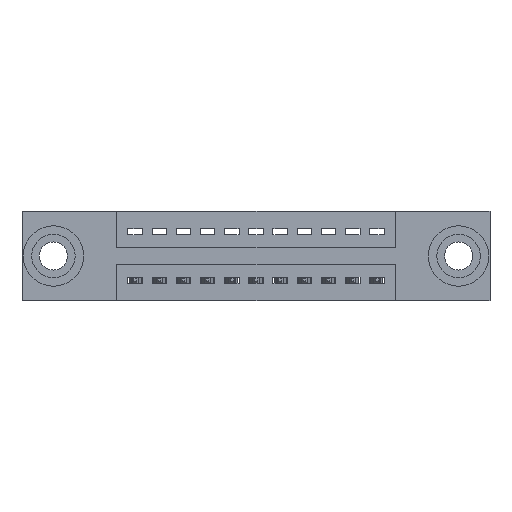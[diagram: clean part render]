
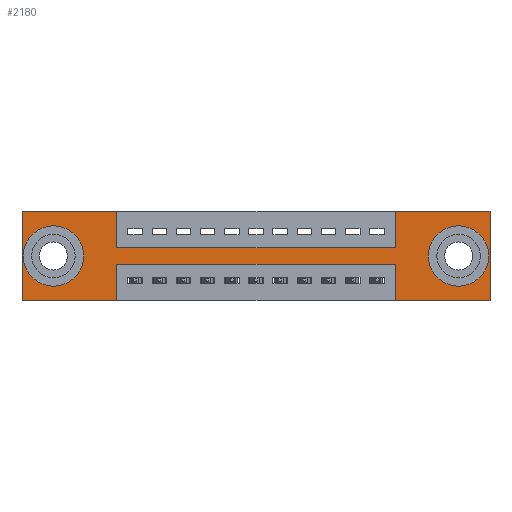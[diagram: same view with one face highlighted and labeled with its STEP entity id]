
A CAD part, front view. The second image highlights one B-rep face of the part: STEP entity #2180.
In plain terms, the highlighted planar face has unit normal (0, -1, 0).
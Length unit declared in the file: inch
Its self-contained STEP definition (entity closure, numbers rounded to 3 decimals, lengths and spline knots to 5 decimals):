
#14 = ORIENTED_EDGE ( 'NONE', *, *, #1394, .T. ) ;
#212 = CARTESIAN_POINT ( 'NONE',  ( 0., 0., 0. ) ) ;
#308 = DIRECTION ( 'NONE',  ( 1., 0., 0. ) ) ;
#668 = EDGE_CURVE ( 'NONE', #12235, #11286, #8197, .T. ) ;
#871 = CARTESIAN_POINT ( 'NONE',  ( 0., 0., 0. ) ) ;
#1046 = CARTESIAN_POINT ( 'NONE',  ( 1.805, 0., -0.185 ) ) ;
#1099 = DIRECTION ( 'NONE',  ( 0., 0., -1. ) ) ;
#1185 = VERTEX_POINT ( 'NONE', #2529 ) ;
#1215 = VERTEX_POINT ( 'NONE', #10645 ) ;
#1394 = EDGE_CURVE ( 'NONE', #10542, #4427, #11053, .T. ) ;
#1672 = VERTEX_POINT ( 'NONE', #3221 ) ;
#1677 = ORIENTED_EDGE ( 'NONE', *, *, #7910, .F. ) ;
#1680 = VERTEX_POINT ( 'NONE', #9301 ) ;
#1684 = EDGE_CURVE ( 'NONE', #12751, #1672, #8982, .T. ) ;
#1815 = DIRECTION ( 'NONE',  ( -1., 0., 0. ) ) ;
#1883 = FACE_BOUND ( 'NONE', #3871, .T. ) ;
#2007 = EDGE_CURVE ( 'NONE', #8037, #3869, #12929, .T. ) ;
#2175 = ORIENTED_EDGE ( 'NONE', *, *, #5121, .F. ) ;
#2180 = ADVANCED_FACE ( 'NONE', ( #1883, #2492, #6230 ), #6213, .T. ) ;
#2492 = FACE_BOUND ( 'NONE', #5449, .T. ) ;
#2529 = CARTESIAN_POINT ( 'NONE',  ( 1.5425, 0., -0.37 ) ) ;
#2872 = VERTEX_POINT ( 'NONE', #11516 ) ;
#2960 = LINE ( 'NONE', #13005, #7366 ) ;
#3043 = LINE ( 'NONE', #7125, #10966 ) ;
#3183 = VECTOR ( 'NONE', #3648, 39.37008 ) ;
#3221 = CARTESIAN_POINT ( 'NONE',  ( 0.3925, 0., 0. ) ) ;
#3309 = CARTESIAN_POINT ( 'NONE',  ( 0., 0., -0.37 ) ) ;
#3332 = DIRECTION ( 'NONE',  ( 0., 0., 1. ) ) ;
#3648 = DIRECTION ( 'NONE',  ( 0., 0., 1. ) ) ;
#3706 = VECTOR ( 'NONE', #9759, 39.37008 ) ;
#3869 = VERTEX_POINT ( 'NONE', #5413 ) ;
#3871 = EDGE_LOOP ( 'NONE', ( #14, #8239 ) ) ;
#4100 = ORIENTED_EDGE ( 'NONE', *, *, #7931, .F. ) ;
#4155 = LINE ( 'NONE', #871, #3706 ) ;
#4224 = DIRECTION ( 'NONE',  ( 1., 0., 0. ) ) ;
#4356 = ORIENTED_EDGE ( 'NONE', *, *, #10420, .F. ) ;
#4414 = ORIENTED_EDGE ( 'NONE', *, *, #11345, .F. ) ;
#4427 = VERTEX_POINT ( 'NONE', #6803 ) ;
#4953 = CARTESIAN_POINT ( 'NONE',  ( 1.805, 0., -0.107 ) ) ;
#5121 = EDGE_CURVE ( 'NONE', #1185, #5389, #6122, .T. ) ;
#5202 = CARTESIAN_POINT ( 'NONE',  ( 0., 0., -0.37 ) ) ;
#5235 = CIRCLE ( 'NONE', #8887, 0.078 ) ;
#5389 = VERTEX_POINT ( 'NONE', #5481 ) ;
#5399 = VERTEX_POINT ( 'NONE', #3309 ) ;
#5413 = CARTESIAN_POINT ( 'NONE',  ( 1.5425, 0., 0. ) ) ;
#5449 = EDGE_LOOP ( 'NONE', ( #11569, #8140 ) ) ;
#5481 = CARTESIAN_POINT ( 'NONE',  ( 1.5425, 0., -0.22 ) ) ;
#5572 = AXIS2_PLACEMENT_3D ( 'NONE', #1046, #8006, #12036 ) ;
#5730 = EDGE_CURVE ( 'NONE', #5399, #12751, #7099, .T. ) ;
#5786 = VECTOR ( 'NONE', #12247, 39.37008 ) ;
#5920 = CARTESIAN_POINT ( 'NONE',  ( 1.935, 0., 0. ) ) ;
#5929 = LINE ( 'NONE', #9885, #6879 ) ;
#5991 = VERTEX_POINT ( 'NONE', #11197 ) ;
#6013 = CARTESIAN_POINT ( 'NONE',  ( 1.5425, 0., -0.15 ) ) ;
#6081 = EDGE_CURVE ( 'NONE', #4427, #10542, #12952, .T. ) ;
#6113 = DIRECTION ( 'NONE',  ( 0., 0., 1. ) ) ;
#6122 = LINE ( 'NONE', #9757, #3183 ) ;
#6207 = LINE ( 'NONE', #5920, #11648 ) ;
#6213 = PLANE ( 'NONE',  #9768 ) ;
#6230 = FACE_OUTER_BOUND ( 'NONE', #8452, .T. ) ;
#6234 = DIRECTION ( 'NONE',  ( 0., 0., -1. ) ) ;
#6285 = DIRECTION ( 'NONE',  ( 0., 1., 0. ) ) ;
#6645 = EDGE_CURVE ( 'NONE', #2872, #8037, #8993, .T. ) ;
#6803 = CARTESIAN_POINT ( 'NONE',  ( 1.805, 0., -0.263 ) ) ;
#6879 = VECTOR ( 'NONE', #8748, 39.37008 ) ;
#6917 = DIRECTION ( 'NONE',  ( -1., 0., 0. ) ) ;
#7029 = VECTOR ( 'NONE', #6917, 39.37008 ) ;
#7099 = LINE ( 'NONE', #8127, #7906 ) ;
#7125 = CARTESIAN_POINT ( 'NONE',  ( 0.3925, 0., 0. ) ) ;
#7149 = CARTESIAN_POINT ( 'NONE',  ( 1.805, 0., -0.185 ) ) ;
#7234 = CARTESIAN_POINT ( 'NONE',  ( 0.3925, 0., -0.15 ) ) ;
#7257 = DIRECTION ( 'NONE',  ( 0., 0., -1. ) ) ;
#7366 = VECTOR ( 'NONE', #1815, 39.37008 ) ;
#7759 = AXIS2_PLACEMENT_3D ( 'NONE', #7149, #10993, #6234 ) ;
#7906 = VECTOR ( 'NONE', #6113, 39.37008 ) ;
#7910 = EDGE_CURVE ( 'NONE', #11834, #5399, #2960, .T. ) ;
#7931 = EDGE_CURVE ( 'NONE', #5389, #5991, #9746, .T. ) ;
#8006 = DIRECTION ( 'NONE',  ( 0., 1., 0. ) ) ;
#8021 = VECTOR ( 'NONE', #308, 39.37008 ) ;
#8037 = VERTEX_POINT ( 'NONE', #6013 ) ;
#8086 = CARTESIAN_POINT ( 'NONE',  ( 0., 0., -0.37 ) ) ;
#8127 = CARTESIAN_POINT ( 'NONE',  ( 0., 0., 0. ) ) ;
#8140 = ORIENTED_EDGE ( 'NONE', *, *, #668, .T. ) ;
#8197 = CIRCLE ( 'NONE', #12876, 0.078 ) ;
#8239 = ORIENTED_EDGE ( 'NONE', *, *, #6081, .T. ) ;
#8273 = CARTESIAN_POINT ( 'NONE',  ( 0., 0., 0. ) ) ;
#8284 = LINE ( 'NONE', #5202, #8777 ) ;
#8409 = CARTESIAN_POINT ( 'NONE',  ( 0.13, 0., -0.185 ) ) ;
#8452 = EDGE_LOOP ( 'NONE', ( #4356, #4100, #2175, #12568, #4414, #11781, #12353, #9204, #8697, #11419, #12489, #1677 ) ) ;
#8485 = CARTESIAN_POINT ( 'NONE',  ( 0.3925, 0., -0.37 ) ) ;
#8697 = ORIENTED_EDGE ( 'NONE', *, *, #12548, .F. ) ;
#8748 = DIRECTION ( 'NONE',  ( 0., 0., -1. ) ) ;
#8777 = VECTOR ( 'NONE', #10359, 39.37008 ) ;
#8875 = CARTESIAN_POINT ( 'NONE',  ( 0.13, 0., -0.107 ) ) ;
#8887 = AXIS2_PLACEMENT_3D ( 'NONE', #10127, #6285, #12432 ) ;
#8982 = LINE ( 'NONE', #8273, #12007 ) ;
#8988 = EDGE_CURVE ( 'NONE', #11286, #12235, #5235, .T. ) ;
#8993 = LINE ( 'NONE', #7234, #8021 ) ;
#9124 = DIRECTION ( 'NONE',  ( 0., -1., 0. ) ) ;
#9204 = ORIENTED_EDGE ( 'NONE', *, *, #6645, .F. ) ;
#9301 = CARTESIAN_POINT ( 'NONE',  ( 1.935, 0., -0.37 ) ) ;
#9746 = LINE ( 'NONE', #13086, #7029 ) ;
#9757 = CARTESIAN_POINT ( 'NONE',  ( 1.5425, 0., -0.37 ) ) ;
#9759 = DIRECTION ( 'NONE',  ( 1., 0., 0. ) ) ;
#9768 = AXIS2_PLACEMENT_3D ( 'NONE', #8086, #9124, #7257 ) ;
#9885 = CARTESIAN_POINT ( 'NONE',  ( 0.3925, 0., -0.37 ) ) ;
#10127 = CARTESIAN_POINT ( 'NONE',  ( 0.13, 0., -0.185 ) ) ;
#10359 = DIRECTION ( 'NONE',  ( -1., 0., 0. ) ) ;
#10420 = EDGE_CURVE ( 'NONE', #5991, #11834, #5929, .T. ) ;
#10542 = VERTEX_POINT ( 'NONE', #4953 ) ;
#10645 = CARTESIAN_POINT ( 'NONE',  ( 1.935, 0., 0. ) ) ;
#10966 = VECTOR ( 'NONE', #1099, 39.37008 ) ;
#10993 = DIRECTION ( 'NONE',  ( 0., 1., 0. ) ) ;
#11053 = CIRCLE ( 'NONE', #5572, 0.078 ) ;
#11082 = DIRECTION ( 'NONE',  ( 0., 0., -1. ) ) ;
#11186 = CARTESIAN_POINT ( 'NONE',  ( 1.5425, 0., 0. ) ) ;
#11197 = CARTESIAN_POINT ( 'NONE',  ( 0.3925, 0., -0.22 ) ) ;
#11259 = EDGE_CURVE ( 'NONE', #3869, #1215, #4155, .T. ) ;
#11286 = VERTEX_POINT ( 'NONE', #8875 ) ;
#11345 = EDGE_CURVE ( 'NONE', #1215, #1680, #6207, .T. ) ;
#11419 = ORIENTED_EDGE ( 'NONE', *, *, #1684, .F. ) ;
#11483 = EDGE_CURVE ( 'NONE', #1680, #1185, #8284, .T. ) ;
#11489 = DIRECTION ( 'NONE',  ( 0., 1., 0. ) ) ;
#11516 = CARTESIAN_POINT ( 'NONE',  ( 0.3925, 0., -0.15 ) ) ;
#11569 = ORIENTED_EDGE ( 'NONE', *, *, #8988, .T. ) ;
#11648 = VECTOR ( 'NONE', #11082, 39.37008 ) ;
#11781 = ORIENTED_EDGE ( 'NONE', *, *, #11259, .F. ) ;
#11834 = VERTEX_POINT ( 'NONE', #8485 ) ;
#12007 = VECTOR ( 'NONE', #4224, 39.37008 ) ;
#12036 = DIRECTION ( 'NONE',  ( 0., 0., -1. ) ) ;
#12235 = VERTEX_POINT ( 'NONE', #13111 ) ;
#12247 = DIRECTION ( 'NONE',  ( 0., 0., 1. ) ) ;
#12353 = ORIENTED_EDGE ( 'NONE', *, *, #2007, .F. ) ;
#12432 = DIRECTION ( 'NONE',  ( 0., 0., 1. ) ) ;
#12489 = ORIENTED_EDGE ( 'NONE', *, *, #5730, .F. ) ;
#12548 = EDGE_CURVE ( 'NONE', #1672, #2872, #3043, .T. ) ;
#12568 = ORIENTED_EDGE ( 'NONE', *, *, #11483, .F. ) ;
#12751 = VERTEX_POINT ( 'NONE', #212 ) ;
#12876 = AXIS2_PLACEMENT_3D ( 'NONE', #8409, #11489, #3332 ) ;
#12929 = LINE ( 'NONE', #11186, #5786 ) ;
#12952 = CIRCLE ( 'NONE', #7759, 0.078 ) ;
#13005 = CARTESIAN_POINT ( 'NONE',  ( 0., 0., -0.37 ) ) ;
#13086 = CARTESIAN_POINT ( 'NONE',  ( 0.3925, 0., -0.22 ) ) ;
#13111 = CARTESIAN_POINT ( 'NONE',  ( 0.13, 0., -0.263 ) ) ;
